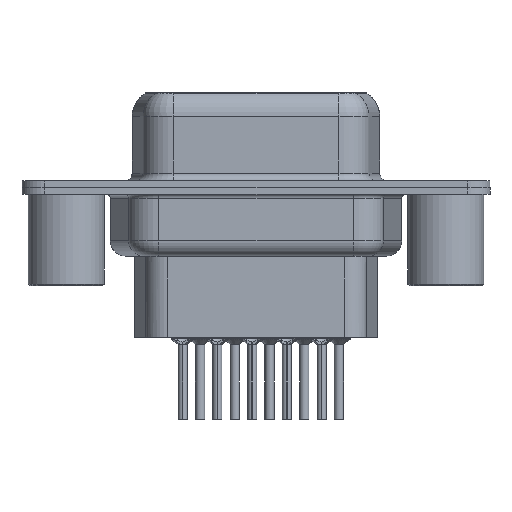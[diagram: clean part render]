
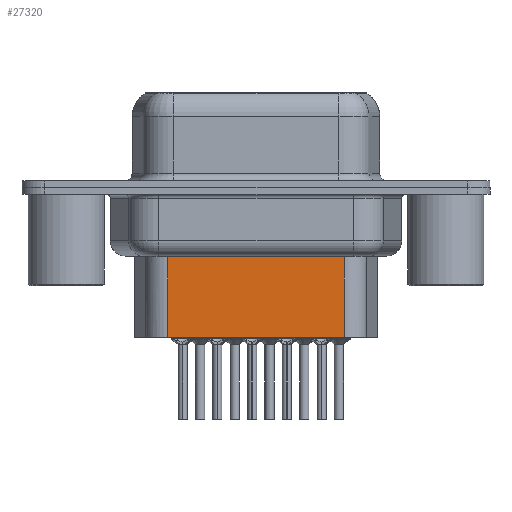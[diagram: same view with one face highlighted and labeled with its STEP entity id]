
A CAD part, front view. The second image highlights one B-rep face of the part: STEP entity #27320.
In plain terms, the highlighted planar face has unit normal (0, -1, 0).
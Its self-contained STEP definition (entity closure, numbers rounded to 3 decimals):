
#278 = ORIENTED_EDGE ( 'NONE', *, *, #1365, .F. ) ;
#982 = VECTOR ( 'NONE', #20936, 1000. ) ;
#1365 = EDGE_CURVE ( 'NONE', #16234, #23689, #20583, .T. ) ;
#3140 = VECTOR ( 'NONE', #28615, 1000. ) ;
#3257 = LINE ( 'NONE', #14081, #19187 ) ;
#3513 = DIRECTION ( 'NONE',  ( 0., -1., 0. ) ) ;
#4810 = VECTOR ( 'NONE', #15904, 1000. ) ;
#5007 = DIRECTION ( 'NONE',  ( -1., 0., 0. ) ) ;
#6588 = EDGE_CURVE ( 'NONE', #23689, #11118, #3257, .T. ) ;
#8588 = LINE ( 'NONE', #15450, #3140 ) ;
#9005 = AXIS2_PLACEMENT_3D ( 'NONE', #19170, #3513, #21663 ) ;
#9770 = CARTESIAN_POINT ( 'NONE',  ( 18.289, -3.5, -4.097 ) ) ;
#9834 = EDGE_LOOP ( 'NONE', ( #278, #26523, #13137, #25849 ) ) ;
#11118 = VERTEX_POINT ( 'NONE', #19202 ) ;
#11517 = VERTEX_POINT ( 'NONE', #18725 ) ;
#12135 = FACE_OUTER_BOUND ( 'NONE', #9834, .T. ) ;
#12283 = CARTESIAN_POINT ( 'NONE',  ( 6.454, -3.5, -4.097 ) ) ;
#13137 = ORIENTED_EDGE ( 'NONE', *, *, #21656, .T. ) ;
#14081 = CARTESIAN_POINT ( 'NONE',  ( 6.701, -3.5, -9.85 ) ) ;
#15450 = CARTESIAN_POINT ( 'NONE',  ( 6.701, -3.5, -3.1 ) ) ;
#15904 = DIRECTION ( 'NONE',  ( 0., 0., -1. ) ) ;
#16234 = VERTEX_POINT ( 'NONE', #9770 ) ;
#17953 = CARTESIAN_POINT ( 'NONE',  ( 18.289, -3.5, -3.1 ) ) ;
#18725 = CARTESIAN_POINT ( 'NONE',  ( 6.701, -3.5, -4.097 ) ) ;
#19170 = CARTESIAN_POINT ( 'NONE',  ( 6.701, -3.5, -3.1 ) ) ;
#19187 = VECTOR ( 'NONE', #5007, 1000. ) ;
#19202 = CARTESIAN_POINT ( 'NONE',  ( 6.701, -3.5, -9.85 ) ) ;
#20583 = LINE ( 'NONE', #17953, #4810 ) ;
#20936 = DIRECTION ( 'NONE',  ( -1., 0., 0. ) ) ;
#21509 = LINE ( 'NONE', #12283, #982 ) ;
#21656 = EDGE_CURVE ( 'NONE', #11517, #11118, #8588, .T. ) ;
#21663 = DIRECTION ( 'NONE',  ( 1., 0., 0. ) ) ;
#23689 = VERTEX_POINT ( 'NONE', #24088 ) ;
#24088 = CARTESIAN_POINT ( 'NONE',  ( 18.289, -3.5, -9.85 ) ) ;
#25849 = ORIENTED_EDGE ( 'NONE', *, *, #6588, .F. ) ;
#26229 = EDGE_CURVE ( 'NONE', #16234, #11517, #21509, .T. ) ;
#26523 = ORIENTED_EDGE ( 'NONE', *, *, #26229, .T. ) ;
#27320 = ADVANCED_FACE ( 'NONE', ( #12135 ), #27650, .T. ) ;
#27650 = PLANE ( 'NONE',  #9005 ) ;
#28615 = DIRECTION ( 'NONE',  ( 0., 0., -1. ) ) ;
